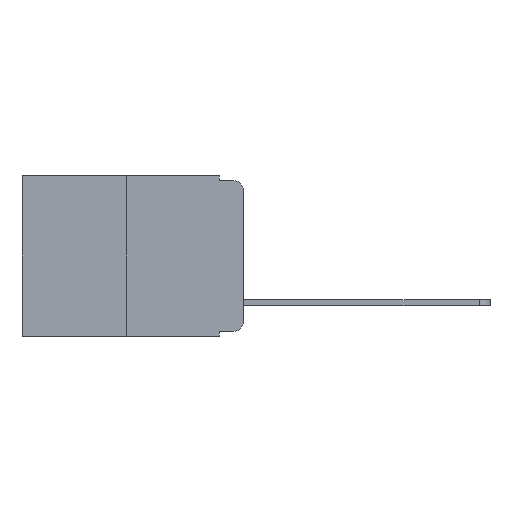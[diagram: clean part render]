
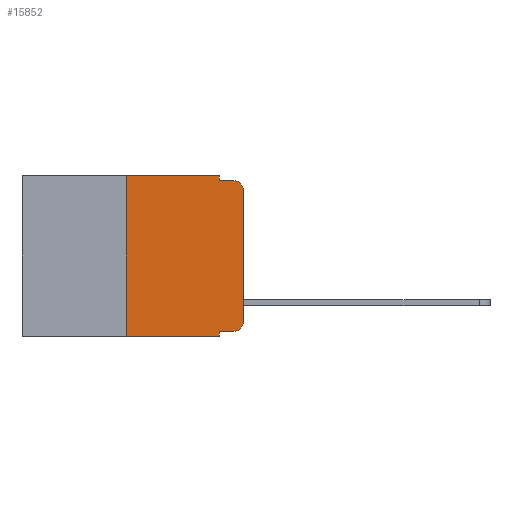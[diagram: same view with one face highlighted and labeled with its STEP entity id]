
A CAD part, left-side view. The second image highlights one B-rep face of the part: STEP entity #15852.
In plain terms, the highlighted planar face has unit normal (-1, 0, 0).
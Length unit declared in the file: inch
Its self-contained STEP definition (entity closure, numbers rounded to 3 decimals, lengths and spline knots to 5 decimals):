
#203 = EDGE_CURVE ( 'NONE', #19027, #1980, #5572, .T. ) ;
#386 = LINE ( 'NONE', #8260, #927 ) ;
#583 = CARTESIAN_POINT ( 'NONE',  ( 0., 0.051, -0.01 ) ) ;
#927 = VECTOR ( 'NONE', #3116, 39.37008 ) ;
#979 = VECTOR ( 'NONE', #20712, 39.37008 ) ;
#995 = DIRECTION ( 'NONE',  ( 0., 0., -1. ) ) ;
#1300 = ORIENTED_EDGE ( 'NONE', *, *, #9399, .T. ) ;
#1344 = LINE ( 'NONE', #8482, #14344 ) ;
#1980 = VERTEX_POINT ( 'NONE', #11784 ) ;
#2315 = DIRECTION ( 'NONE',  ( 0., 0., -1. ) ) ;
#2385 = ORIENTED_EDGE ( 'NONE', *, *, #7135, .F. ) ;
#2531 = EDGE_CURVE ( 'NONE', #19027, #3573, #3629, .T. ) ;
#2836 = EDGE_CURVE ( 'NONE', #6414, #3573, #11317, .T. ) ;
#3047 = VECTOR ( 'NONE', #16232, 39.37008 ) ;
#3116 = DIRECTION ( 'NONE',  ( 0., -1., 0. ) ) ;
#3162 = AXIS2_PLACEMENT_3D ( 'NONE', #20690, #12461, #2315 ) ;
#3239 = CARTESIAN_POINT ( 'NONE',  ( 0., 0.473, 0. ) ) ;
#3573 = VERTEX_POINT ( 'NONE', #19780 ) ;
#3629 = LINE ( 'NONE', #8221, #20873 ) ;
#3701 = EDGE_CURVE ( 'NONE', #6414, #3847, #16201, .T. ) ;
#3847 = VERTEX_POINT ( 'NONE', #7545 ) ;
#3899 = VERTEX_POINT ( 'NONE', #6912 ) ;
#4450 = CIRCLE ( 'NONE', #18655, 0.02 ) ;
#4821 = DIRECTION ( 'NONE',  ( 0., 0., 1. ) ) ;
#4855 = EDGE_CURVE ( 'NONE', #10438, #18674, #1344, .T. ) ;
#5301 = CARTESIAN_POINT ( 'NONE',  ( 0., 0.02, -0.01 ) ) ;
#5572 = LINE ( 'NONE', #12205, #979 ) ;
#5897 = EDGE_LOOP ( 'NONE', ( #1300, #15330, #2385, #11968, #16887, #17395, #21780, #9609, #10659, #15082 ) ) ;
#6414 = VERTEX_POINT ( 'NONE', #16308 ) ;
#6912 = CARTESIAN_POINT ( 'NONE',  ( 0., 0., -0.03 ) ) ;
#7135 = EDGE_CURVE ( 'NONE', #18674, #9694, #386, .T. ) ;
#7350 = VECTOR ( 'NONE', #16780, 39.37008 ) ;
#7545 = CARTESIAN_POINT ( 'NONE',  ( 0., 0.25, 0. ) ) ;
#7783 = CARTESIAN_POINT ( 'NONE',  ( 0., 0., -0.313 ) ) ;
#8162 = CARTESIAN_POINT ( 'NONE',  ( 0., 0.02, -0.313 ) ) ;
#8221 = CARTESIAN_POINT ( 'NONE',  ( 0., 0.051, 0. ) ) ;
#8260 = CARTESIAN_POINT ( 'NONE',  ( 0., 0.051, -0.01 ) ) ;
#8270 = EDGE_CURVE ( 'NONE', #3899, #9694, #4450, .T. ) ;
#8482 = CARTESIAN_POINT ( 'NONE',  ( 0., 0.051, 0. ) ) ;
#9345 = CARTESIAN_POINT ( 'NONE',  ( 0., 0.25, 0. ) ) ;
#9399 = EDGE_CURVE ( 'NONE', #20793, #3899, #16459, .T. ) ;
#9609 = ORIENTED_EDGE ( 'NONE', *, *, #2531, .F. ) ;
#9694 = VERTEX_POINT ( 'NONE', #5301 ) ;
#9875 = DIRECTION ( 'NONE',  ( 0., 0., -1. ) ) ;
#9917 = DIRECTION ( 'NONE',  ( -1., 0., 0. ) ) ;
#9918 = CIRCLE ( 'NONE', #20727, 0.02 ) ;
#10438 = VERTEX_POINT ( 'NONE', #19286 ) ;
#10659 = ORIENTED_EDGE ( 'NONE', *, *, #203, .T. ) ;
#10684 = EDGE_CURVE ( 'NONE', #3847, #10438, #11483, .T. ) ;
#11317 = LINE ( 'NONE', #19535, #7350 ) ;
#11483 = LINE ( 'NONE', #3239, #16398 ) ;
#11784 = CARTESIAN_POINT ( 'NONE',  ( 0., 0.02, -0.333 ) ) ;
#11968 = ORIENTED_EDGE ( 'NONE', *, *, #4855, .F. ) ;
#12205 = CARTESIAN_POINT ( 'NONE',  ( 0., 0.051, -0.333 ) ) ;
#12461 = DIRECTION ( 'NONE',  ( 1., 0., 0. ) ) ;
#12894 = CARTESIAN_POINT ( 'NONE',  ( 0., 0., 0. ) ) ;
#14344 = VECTOR ( 'NONE', #20073, 39.37008 ) ;
#15082 = ORIENTED_EDGE ( 'NONE', *, *, #20904, .T. ) ;
#15173 = VECTOR ( 'NONE', #4821, 39.37008 ) ;
#15330 = ORIENTED_EDGE ( 'NONE', *, *, #8270, .T. ) ;
#15852 = ADVANCED_FACE ( 'NONE', ( #16725 ), #19061, .F. ) ;
#16201 = LINE ( 'NONE', #9345, #15173 ) ;
#16232 = DIRECTION ( 'NONE',  ( 0., 0., 1. ) ) ;
#16308 = CARTESIAN_POINT ( 'NONE',  ( 0., 0.25, -0.343 ) ) ;
#16398 = VECTOR ( 'NONE', #16689, 39.37008 ) ;
#16459 = LINE ( 'NONE', #12894, #3047 ) ;
#16689 = DIRECTION ( 'NONE',  ( 0., -1., 0. ) ) ;
#16725 = FACE_OUTER_BOUND ( 'NONE', #5897, .T. ) ;
#16780 = DIRECTION ( 'NONE',  ( 0., -1., 0. ) ) ;
#16887 = ORIENTED_EDGE ( 'NONE', *, *, #10684, .F. ) ;
#17395 = ORIENTED_EDGE ( 'NONE', *, *, #3701, .F. ) ;
#18655 = AXIS2_PLACEMENT_3D ( 'NONE', #19824, #9917, #21493 ) ;
#18674 = VERTEX_POINT ( 'NONE', #583 ) ;
#19027 = VERTEX_POINT ( 'NONE', #20138 ) ;
#19061 = PLANE ( 'NONE',  #3162 ) ;
#19286 = CARTESIAN_POINT ( 'NONE',  ( 0., 0.051, 0. ) ) ;
#19535 = CARTESIAN_POINT ( 'NONE',  ( 0., 0.473, -0.343 ) ) ;
#19780 = CARTESIAN_POINT ( 'NONE',  ( 0., 0.051, -0.343 ) ) ;
#19784 = DIRECTION ( 'NONE',  ( -1., 0., 0. ) ) ;
#19824 = CARTESIAN_POINT ( 'NONE',  ( 0., 0.02, -0.03 ) ) ;
#20073 = DIRECTION ( 'NONE',  ( 0., 0., -1. ) ) ;
#20138 = CARTESIAN_POINT ( 'NONE',  ( 0., 0.051, -0.333 ) ) ;
#20690 = CARTESIAN_POINT ( 'NONE',  ( 0., 0.473, 0. ) ) ;
#20712 = DIRECTION ( 'NONE',  ( 0., -1., 0. ) ) ;
#20727 = AXIS2_PLACEMENT_3D ( 'NONE', #8162, #19784, #9875 ) ;
#20793 = VERTEX_POINT ( 'NONE', #7783 ) ;
#20873 = VECTOR ( 'NONE', #995, 39.37008 ) ;
#20904 = EDGE_CURVE ( 'NONE', #1980, #20793, #9918, .T. ) ;
#21493 = DIRECTION ( 'NONE',  ( 0., 0., -1. ) ) ;
#21780 = ORIENTED_EDGE ( 'NONE', *, *, #2836, .T. ) ;
